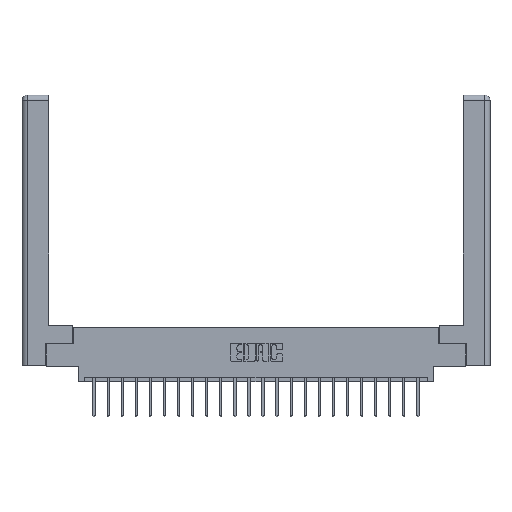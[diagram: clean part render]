
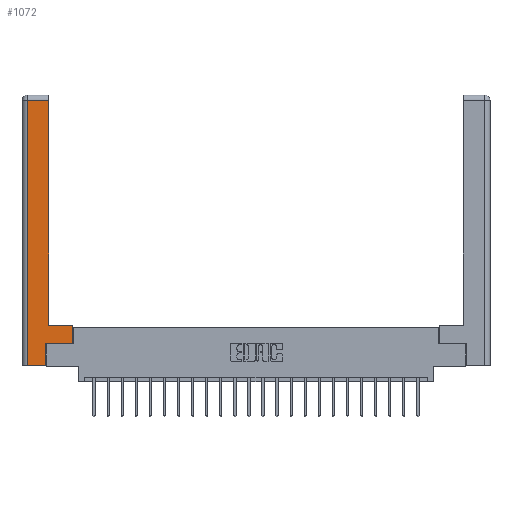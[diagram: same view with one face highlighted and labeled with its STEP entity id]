
A CAD part, top view. The second image highlights one B-rep face of the part: STEP entity #1072.
In plain terms, the highlighted planar face has unit normal (0, 0, 1).
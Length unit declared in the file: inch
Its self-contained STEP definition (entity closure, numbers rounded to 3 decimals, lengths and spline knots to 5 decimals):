
#15 = PLANE ( 'NONE',  #23366 ) ;
#753 = CARTESIAN_POINT ( 'NONE',  ( 0.565, 0.245, 0. ) ) ;
#1072 = ADVANCED_FACE ( 'NONE', ( #17004 ), #15, .F. ) ;
#1410 = VECTOR ( 'NONE', #17727, 39.37008 ) ;
#2149 = VERTEX_POINT ( 'NONE', #18653 ) ;
#2253 = CARTESIAN_POINT ( 'NONE',  ( 0.265, 0.245, 0. ) ) ;
#2309 = VERTEX_POINT ( 'NONE', #17475 ) ;
#3197 = VERTEX_POINT ( 'NONE', #7596 ) ;
#3410 = EDGE_CURVE ( 'NONE', #22091, #6557, #9280, .T. ) ;
#3459 = CARTESIAN_POINT ( 'NONE',  ( 0., 0., 0. ) ) ;
#3996 = CARTESIAN_POINT ( 'NONE',  ( 0.0615, 2.94, 0. ) ) ;
#5018 = DIRECTION ( 'NONE',  ( 0., 1., 0. ) ) ;
#5981 = EDGE_CURVE ( 'NONE', #20396, #22091, #11437, .T. ) ;
#6270 = VECTOR ( 'NONE', #23444, 39.37008 ) ;
#6557 = VERTEX_POINT ( 'NONE', #16594 ) ;
#6727 = CARTESIAN_POINT ( 'NONE',  ( 0.295, 0.45, 0. ) ) ;
#6820 = CARTESIAN_POINT ( 'NONE',  ( 0.0615, 0., 0. ) ) ;
#7087 = CARTESIAN_POINT ( 'NONE',  ( 0.265, 0., 0. ) ) ;
#7134 = DIRECTION ( 'NONE',  ( -1., 0., 0. ) ) ;
#7320 = LINE ( 'NONE', #6727, #17038 ) ;
#7596 = CARTESIAN_POINT ( 'NONE',  ( 0.265, 0., 0. ) ) ;
#7930 = VECTOR ( 'NONE', #13537, 39.37008 ) ;
#8095 = VECTOR ( 'NONE', #8647, 39.37008 ) ;
#8647 = DIRECTION ( 'NONE',  ( 0., -1., 0. ) ) ;
#9067 = CARTESIAN_POINT ( 'NONE',  ( 0.295, 2.94, 0. ) ) ;
#9280 = LINE ( 'NONE', #3996, #15022 ) ;
#9686 = EDGE_CURVE ( 'NONE', #12580, #2149, #20870, .T. ) ;
#10409 = DIRECTION ( 'NONE',  ( -1., 0., 0. ) ) ;
#10757 = DIRECTION ( 'NONE',  ( 0., 1., 0. ) ) ;
#10899 = EDGE_CURVE ( 'NONE', #2149, #20396, #7320, .T. ) ;
#11437 = LINE ( 'NONE', #18345, #12574 ) ;
#11589 = CARTESIAN_POINT ( 'NONE',  ( 0.565, 0.245, 0. ) ) ;
#12109 = CARTESIAN_POINT ( 'NONE',  ( 0.265, 0.245, 0. ) ) ;
#12460 = ORIENTED_EDGE ( 'NONE', *, *, #10899, .T. ) ;
#12574 = VECTOR ( 'NONE', #10757, 39.37008 ) ;
#12580 = VERTEX_POINT ( 'NONE', #753 ) ;
#13047 = VERTEX_POINT ( 'NONE', #2253 ) ;
#13074 = DIRECTION ( 'NONE',  ( -1., 0., 0. ) ) ;
#13126 = LINE ( 'NONE', #7087, #6270 ) ;
#13303 = ORIENTED_EDGE ( 'NONE', *, *, #19008, .T. ) ;
#13537 = DIRECTION ( 'NONE',  ( 1., 0., 0. ) ) ;
#13935 = ORIENTED_EDGE ( 'NONE', *, *, #9686, .T. ) ;
#14003 = LINE ( 'NONE', #12109, #1410 ) ;
#14383 = ORIENTED_EDGE ( 'NONE', *, *, #3410, .T. ) ;
#15022 = VECTOR ( 'NONE', #13074, 39.37008 ) ;
#16217 = DIRECTION ( 'NONE',  ( 0., 0., -1. ) ) ;
#16594 = CARTESIAN_POINT ( 'NONE',  ( 0.0615, 2.94, 0. ) ) ;
#16958 = LINE ( 'NONE', #6820, #8095 ) ;
#17004 = FACE_OUTER_BOUND ( 'NONE', #17801, .T. ) ;
#17038 = VECTOR ( 'NONE', #10409, 39.37008 ) ;
#17199 = ORIENTED_EDGE ( 'NONE', *, *, #21438, .T. ) ;
#17233 = ORIENTED_EDGE ( 'NONE', *, *, #5981, .T. ) ;
#17475 = CARTESIAN_POINT ( 'NONE',  ( 0.0615, 0., 0. ) ) ;
#17723 = EDGE_CURVE ( 'NONE', #2309, #3197, #13126, .T. ) ;
#17727 = DIRECTION ( 'NONE',  ( 0., 1., 0. ) ) ;
#17801 = EDGE_LOOP ( 'NONE', ( #17233, #14383, #17199, #22670, #21286, #13303, #13935, #12460 ) ) ;
#18230 = LINE ( 'NONE', #11589, #7930 ) ;
#18345 = CARTESIAN_POINT ( 'NONE',  ( 0.295, 3., 0. ) ) ;
#18653 = CARTESIAN_POINT ( 'NONE',  ( 0.565, 0.45, 0. ) ) ;
#19008 = EDGE_CURVE ( 'NONE', #13047, #12580, #18230, .T. ) ;
#20396 = VERTEX_POINT ( 'NONE', #23445 ) ;
#20498 = EDGE_CURVE ( 'NONE', #3197, #13047, #14003, .T. ) ;
#20592 = VECTOR ( 'NONE', #5018, 39.37008 ) ;
#20870 = LINE ( 'NONE', #22669, #20592 ) ;
#21286 = ORIENTED_EDGE ( 'NONE', *, *, #20498, .T. ) ;
#21438 = EDGE_CURVE ( 'NONE', #6557, #2309, #16958, .T. ) ;
#22091 = VERTEX_POINT ( 'NONE', #9067 ) ;
#22669 = CARTESIAN_POINT ( 'NONE',  ( 0.565, 0.45, 0. ) ) ;
#22670 = ORIENTED_EDGE ( 'NONE', *, *, #17723, .T. ) ;
#23366 = AXIS2_PLACEMENT_3D ( 'NONE', #3459, #16217, #7134 ) ;
#23444 = DIRECTION ( 'NONE',  ( 1., 0., 0. ) ) ;
#23445 = CARTESIAN_POINT ( 'NONE',  ( 0.295, 0.45, 0. ) ) ;
